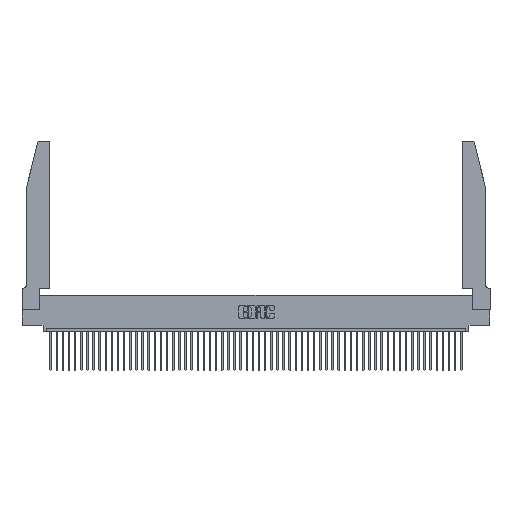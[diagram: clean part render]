
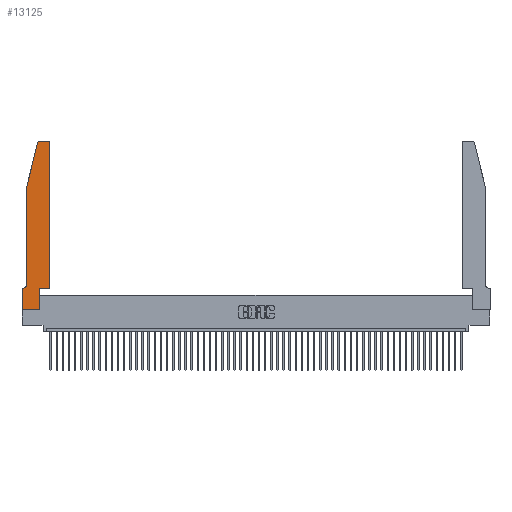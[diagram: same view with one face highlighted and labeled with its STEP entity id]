
A CAD part, top view. The second image highlights one B-rep face of the part: STEP entity #13125.
In plain terms, the highlighted planar face has unit normal (0, 0, 1).
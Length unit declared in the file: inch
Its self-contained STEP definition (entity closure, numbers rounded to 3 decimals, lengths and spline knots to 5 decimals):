
#2688 = VECTOR ( 'NONE', #42561, 39.37008 ) ;
#3496 = EDGE_LOOP ( 'NONE', ( #49750, #44035, #43782, #38057, #5638, #8652, #4046, #6966, #7066, #8179, #25272, #48598 ) ) ;
#4046 = ORIENTED_EDGE ( 'NONE', *, *, #11160, .T. ) ;
#4442 = FACE_OUTER_BOUND ( 'NONE', #3496, .T. ) ;
#5140 = CARTESIAN_POINT ( 'NONE',  ( 0.2865, 0., 0.37 ) ) ;
#5638 = ORIENTED_EDGE ( 'NONE', *, *, #13195, .T. ) ;
#6120 = EDGE_CURVE ( 'NONE', #26238, #7433, #50296, .T. ) ;
#6727 = EDGE_CURVE ( 'NONE', #15881, #22715, #14732, .T. ) ;
#6966 = ORIENTED_EDGE ( 'NONE', *, *, #20365, .T. ) ;
#7066 = ORIENTED_EDGE ( 'NONE', *, *, #6120, .T. ) ;
#7433 = VERTEX_POINT ( 'NONE', #40537 ) ;
#7577 = DIRECTION ( 'NONE',  ( 1., 0., 0. ) ) ;
#7707 = VECTOR ( 'NONE', #39176, 39.37008 ) ;
#8179 = ORIENTED_EDGE ( 'NONE', *, *, #44811, .T. ) ;
#8652 = ORIENTED_EDGE ( 'NONE', *, *, #21169, .T. ) ;
#9380 = CARTESIAN_POINT ( 'NONE',  ( 0.0755, 0.42, 0.37 ) ) ;
#9632 = CARTESIAN_POINT ( 'NONE',  ( 0., 0., 0.37 ) ) ;
#9709 = VECTOR ( 'NONE', #15550, 39.37008 ) ;
#10065 = CARTESIAN_POINT ( 'NONE',  ( 0., 0.35, 0.37 ) ) ;
#10189 = AXIS2_PLACEMENT_3D ( 'NONE', #27525, #39783, #7577 ) ;
#10720 = DIRECTION ( 'NONE',  ( -1., 0., 0. ) ) ;
#10841 = LINE ( 'NONE', #21361, #7707 ) ;
#11109 = VERTEX_POINT ( 'NONE', #48984 ) ;
#11160 = EDGE_CURVE ( 'NONE', #14866, #48781, #23179, .T. ) ;
#11564 = CARTESIAN_POINT ( 'NONE',  ( 0.4505, 0.35, 0.37 ) ) ;
#11720 = VECTOR ( 'NONE', #34208, 39.37008 ) ;
#12326 = CIRCLE ( 'NONE', #32442, 0.03 ) ;
#12363 = EDGE_CURVE ( 'NONE', #22715, #20368, #26728, .T. ) ;
#13125 = ADVANCED_FACE ( 'NONE', ( #4442 ), #44263, .T. ) ;
#13195 = EDGE_CURVE ( 'NONE', #26593, #11109, #46949, .T. ) ;
#13517 = CARTESIAN_POINT ( 'NONE',  ( 0.284, 2.75, 0.37 ) ) ;
#14010 = CARTESIAN_POINT ( 'NONE',  ( 0.25487, 2.72718, 0.37 ) ) ;
#14732 = LINE ( 'NONE', #14760, #2688 ) ;
#14760 = CARTESIAN_POINT ( 'NONE',  ( 0.4505, 0.35, 0.37 ) ) ;
#14866 = VERTEX_POINT ( 'NONE', #10065 ) ;
#15550 = DIRECTION ( 'NONE',  ( 0., 1., 0. ) ) ;
#15599 = VECTOR ( 'NONE', #46771, 39.37008 ) ;
#15672 = AXIS2_PLACEMENT_3D ( 'NONE', #35444, #51871, #51328 ) ;
#15881 = VERTEX_POINT ( 'NONE', #44917 ) ;
#18504 = LINE ( 'NONE', #42780, #22286 ) ;
#19411 = EDGE_CURVE ( 'NONE', #29371, #21150, #12326, .T. ) ;
#20365 = EDGE_CURVE ( 'NONE', #48781, #26238, #28057, .T. ) ;
#20368 = VERTEX_POINT ( 'NONE', #29922 ) ;
#20416 = DIRECTION ( 'NONE',  ( 0., -1., 0. ) ) ;
#20675 = DIRECTION ( 'NONE',  ( 0., 0., 1. ) ) ;
#20840 = DIRECTION ( 'NONE',  ( 1., 0., 0. ) ) ;
#21150 = VERTEX_POINT ( 'NONE', #14010 ) ;
#21169 = EDGE_CURVE ( 'NONE', #11109, #14866, #18504, .T. ) ;
#21361 = CARTESIAN_POINT ( 'NONE',  ( 0.0755, 2., 0.37 ) ) ;
#22286 = VECTOR ( 'NONE', #10720, 39.37008 ) ;
#22715 = VERTEX_POINT ( 'NONE', #25416 ) ;
#23179 = LINE ( 'NONE', #30554, #15599 ) ;
#25098 = DIRECTION ( 'NONE',  ( -1., 0., 0. ) ) ;
#25254 = VECTOR ( 'NONE', #31693, 39.37008 ) ;
#25272 = ORIENTED_EDGE ( 'NONE', *, *, #6727, .T. ) ;
#25416 = CARTESIAN_POINT ( 'NONE',  ( 0.4505, 2.72, 0.37 ) ) ;
#25970 = CARTESIAN_POINT ( 'NONE',  ( 0.0755, 2., 0.37 ) ) ;
#26238 = VERTEX_POINT ( 'NONE', #5140 ) ;
#26593 = VERTEX_POINT ( 'NONE', #9380 ) ;
#26728 = CIRCLE ( 'NONE', #36607, 0.03 ) ;
#27525 = CARTESIAN_POINT ( 'NONE',  ( 0., 0.35, 0.37 ) ) ;
#28057 = LINE ( 'NONE', #9632, #11720 ) ;
#28808 = CARTESIAN_POINT ( 'NONE',  ( 0.2605, 2.75, 0.37 ) ) ;
#28847 = VECTOR ( 'NONE', #20416, 39.37008 ) ;
#29371 = VERTEX_POINT ( 'NONE', #13517 ) ;
#29922 = CARTESIAN_POINT ( 'NONE',  ( 0.4205, 2.75, 0.37 ) ) ;
#30291 = CARTESIAN_POINT ( 'NONE',  ( 0., 0., 0.37 ) ) ;
#30554 = CARTESIAN_POINT ( 'NONE',  ( 0., 0., 0.37 ) ) ;
#31128 = EDGE_CURVE ( 'NONE', #21150, #44579, #10841, .T. ) ;
#31693 = DIRECTION ( 'NONE',  ( 1., 0., 0. ) ) ;
#32442 = AXIS2_PLACEMENT_3D ( 'NONE', #45030, #20675, #20840 ) ;
#34208 = DIRECTION ( 'NONE',  ( 1., 0., 0. ) ) ;
#35444 = CARTESIAN_POINT ( 'NONE',  ( 0.0055, 0.42, 0.37 ) ) ;
#36570 = CARTESIAN_POINT ( 'NONE',  ( 0.4205, 2.72, 0.37 ) ) ;
#36607 = AXIS2_PLACEMENT_3D ( 'NONE', #36570, #40676, #49684 ) ;
#36670 = LINE ( 'NONE', #11564, #25254 ) ;
#36946 = EDGE_CURVE ( 'NONE', #20368, #29371, #51224, .T. ) ;
#38057 = ORIENTED_EDGE ( 'NONE', *, *, #46595, .T. ) ;
#39176 = DIRECTION ( 'NONE',  ( -0.239, -0.971, 0. ) ) ;
#39767 = LINE ( 'NONE', #48544, #28847 ) ;
#39783 = DIRECTION ( 'NONE',  ( 0., 0., 1. ) ) ;
#40537 = CARTESIAN_POINT ( 'NONE',  ( 0.2865, 0.35, 0.37 ) ) ;
#40676 = DIRECTION ( 'NONE',  ( 0., 0., 1. ) ) ;
#42561 = DIRECTION ( 'NONE',  ( 0., 1., 0. ) ) ;
#42780 = CARTESIAN_POINT ( 'NONE',  ( 0.0755, 0.35, 0.37 ) ) ;
#43764 = CARTESIAN_POINT ( 'NONE',  ( 0.2865, 0.35, 0.37 ) ) ;
#43782 = ORIENTED_EDGE ( 'NONE', *, *, #31128, .T. ) ;
#44035 = ORIENTED_EDGE ( 'NONE', *, *, #19411, .T. ) ;
#44263 = PLANE ( 'NONE',  #10189 ) ;
#44579 = VERTEX_POINT ( 'NONE', #25970 ) ;
#44811 = EDGE_CURVE ( 'NONE', #7433, #15881, #36670, .T. ) ;
#44917 = CARTESIAN_POINT ( 'NONE',  ( 0.4505, 0.35, 0.37 ) ) ;
#45030 = CARTESIAN_POINT ( 'NONE',  ( 0.284, 2.72, 0.37 ) ) ;
#45307 = VECTOR ( 'NONE', #25098, 39.37008 ) ;
#46595 = EDGE_CURVE ( 'NONE', #44579, #26593, #39767, .T. ) ;
#46771 = DIRECTION ( 'NONE',  ( 0., -1., 0. ) ) ;
#46949 = CIRCLE ( 'NONE', #15672, 0.07 ) ;
#48544 = CARTESIAN_POINT ( 'NONE',  ( 0.0755, 2., 0.37 ) ) ;
#48598 = ORIENTED_EDGE ( 'NONE', *, *, #12363, .T. ) ;
#48781 = VERTEX_POINT ( 'NONE', #30291 ) ;
#48984 = CARTESIAN_POINT ( 'NONE',  ( 0.0055, 0.35, 0.37 ) ) ;
#49684 = DIRECTION ( 'NONE',  ( 1., 0., 0. ) ) ;
#49750 = ORIENTED_EDGE ( 'NONE', *, *, #36946, .T. ) ;
#50296 = LINE ( 'NONE', #43764, #9709 ) ;
#51224 = LINE ( 'NONE', #28808, #45307 ) ;
#51328 = DIRECTION ( 'NONE',  ( -1., 0., 0. ) ) ;
#51871 = DIRECTION ( 'NONE',  ( 0., 0., -1. ) ) ;
